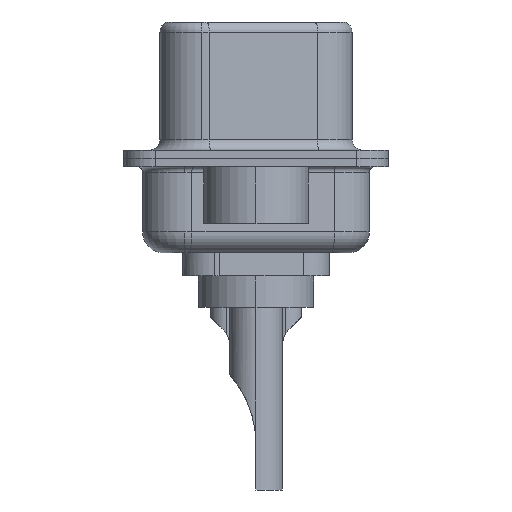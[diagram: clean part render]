
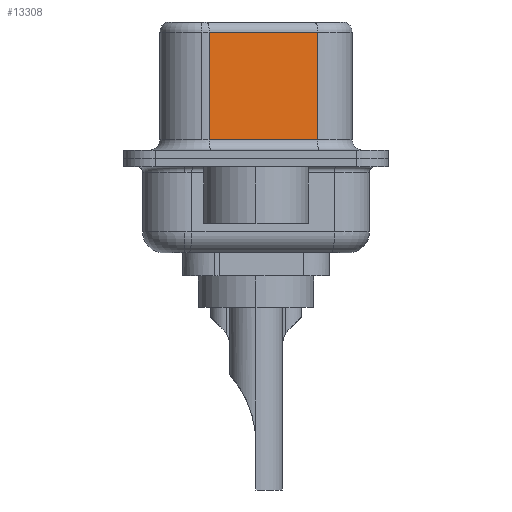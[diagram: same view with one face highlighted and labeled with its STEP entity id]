
A CAD part, left-side view. The second image highlights one B-rep face of the part: STEP entity #13308.
In plain terms, the highlighted planar face has unit normal (-0.985, -0.174, 0).
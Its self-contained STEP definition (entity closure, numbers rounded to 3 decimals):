
#988 = VERTEX_POINT ( 'NONE', #9394 ) ;
#1782 = ORIENTED_EDGE ( 'NONE', *, *, #13832, .F. ) ;
#2245 = ORIENTED_EDGE ( 'NONE', *, *, #12284, .T. ) ;
#2455 = LINE ( 'NONE', #17217, #2903 ) ;
#2600 = EDGE_LOOP ( 'NONE', ( #1782, #2245, #17997, #14568 ) ) ;
#2903 = VECTOR ( 'NONE', #18578, 1000. ) ;
#2905 = CARTESIAN_POINT ( 'NONE',  ( 3.675, 2.233, 6.52 ) ) ;
#4076 = PLANE ( 'NONE',  #11942 ) ;
#4327 = DIRECTION ( 'NONE',  ( 0., 0., -1. ) ) ;
#4606 = CARTESIAN_POINT ( 'NONE',  ( 3.675, 2.233, 6.02 ) ) ;
#5363 = CARTESIAN_POINT ( 'NONE',  ( 4.585, -2.927, 6.02 ) ) ;
#5593 = EDGE_CURVE ( 'NONE', #988, #6052, #6967, .T. ) ;
#6052 = VERTEX_POINT ( 'NONE', #17231 ) ;
#6679 = VERTEX_POINT ( 'NONE', #11606 ) ;
#6967 = LINE ( 'NONE', #8406, #17864 ) ;
#7632 = VECTOR ( 'NONE', #4327, 1000. ) ;
#8406 = CARTESIAN_POINT ( 'NONE',  ( 4.585, -2.927, 0.9 ) ) ;
#8523 = DIRECTION ( 'NONE',  ( 0.985, 0.174, 0. ) ) ;
#8944 = VECTOR ( 'NONE', #13942, 1000. ) ;
#9394 = CARTESIAN_POINT ( 'NONE',  ( 3.675, 2.233, 0.9 ) ) ;
#9794 = FACE_OUTER_BOUND ( 'NONE', #2600, .T. ) ;
#9824 = LINE ( 'NONE', #5363, #8944 ) ;
#10131 = EDGE_CURVE ( 'NONE', #17542, #988, #15102, .T. ) ;
#11280 = CARTESIAN_POINT ( 'NONE',  ( 4.585, -2.927, 6.52 ) ) ;
#11606 = CARTESIAN_POINT ( 'NONE',  ( 4.585, -2.927, 6.02 ) ) ;
#11942 = AXIS2_PLACEMENT_3D ( 'NONE', #11280, #8523, #18394 ) ;
#12284 = EDGE_CURVE ( 'NONE', #6679, #17542, #9824, .T. ) ;
#12364 = DIRECTION ( 'NONE',  ( 0.174, -0.985, 0. ) ) ;
#13308 = ADVANCED_FACE ( 'NONE', ( #9794 ), #4076, .F. ) ;
#13832 = EDGE_CURVE ( 'NONE', #6679, #6052, #2455, .T. ) ;
#13942 = DIRECTION ( 'NONE',  ( -0.174, 0.985, 0. ) ) ;
#14568 = ORIENTED_EDGE ( 'NONE', *, *, #5593, .T. ) ;
#15102 = LINE ( 'NONE', #2905, #7632 ) ;
#17217 = CARTESIAN_POINT ( 'NONE',  ( 4.585, -2.927, 6.52 ) ) ;
#17231 = CARTESIAN_POINT ( 'NONE',  ( 4.585, -2.927, 0.9 ) ) ;
#17542 = VERTEX_POINT ( 'NONE', #4606 ) ;
#17864 = VECTOR ( 'NONE', #12364, 1000. ) ;
#17997 = ORIENTED_EDGE ( 'NONE', *, *, #10131, .T. ) ;
#18394 = DIRECTION ( 'NONE',  ( -0.174, 0.985, 0. ) ) ;
#18578 = DIRECTION ( 'NONE',  ( 0., 0., -1. ) ) ;
